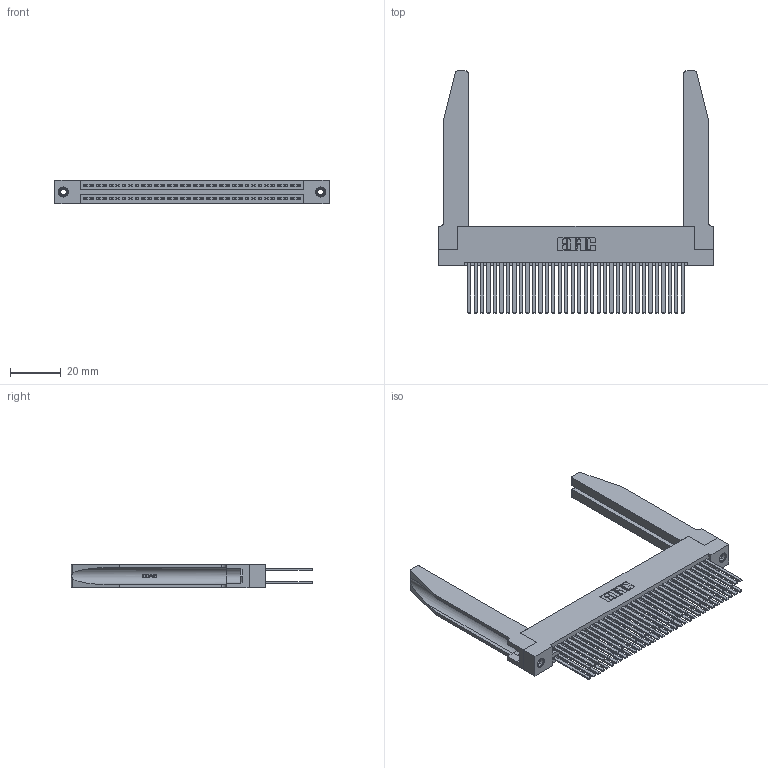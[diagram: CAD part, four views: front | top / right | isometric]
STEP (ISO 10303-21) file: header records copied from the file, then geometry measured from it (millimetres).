
FILE_DESCRIPTION (( 'STEP AP203' ), '1' );
FILE_NAME ('395-068-544-278.STEP', '2019-10-23T23:06:55', ( '' ), ( '' ), 'SwSTEP 2.0', 'SolidWorks 2016', '' );
FILE_SCHEMA (( 'CONFIG_CONTROL_DESIGN' ));
Length unit declared in the file: inch
Products named in the file (5): 345-250-001_345-250-001-102; 345-220-078_345-220-078; 395-068-544-278; 345 Part_Flush Mounting Lugs - 0.156 Dia-TH; 345-292-001_345-293-144
Assembly tree (73 placements, depth 2):
  395-068-544-278
    345 Part_Flush Mounting Lugs - 0.156 Dia-TH
    345-292-001_345-293-144  x68
    345-250-001_345-250-001-102  x2
    345-220-078_345-220-078  x2
Bounding box: 107.59 x 94.92 x 9.4 mm (x, y, z)
Volume: 19101.2 mm3; surface area: 26226.2 mm2
Topology: 73 solids, 73 shells, 3352 faces, 9857 edges, 6470 vertices
Faces by surface type: plane 2194, cylinder 1106, bspline 36, cone 12, torus 4
Entity records: 32310 total; most frequent: CARTESIAN_POINT 6339, ORIENTED_EDGE 5170, DIRECTION 4591, EDGE_CURVE 2585, VECTOR 2227, LINE 2227, VERTEX_POINT 1716, AXIS2_PLACEMENT_3D 1182
